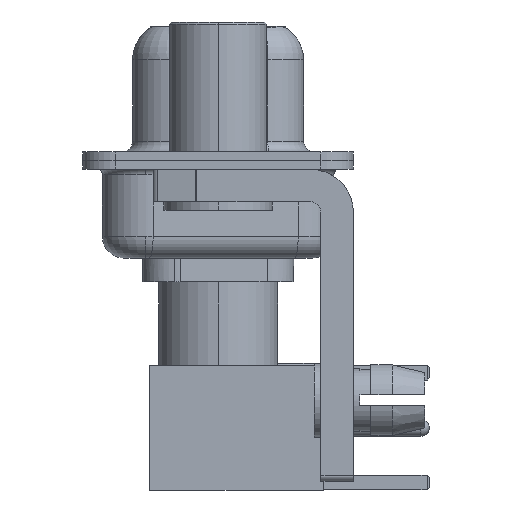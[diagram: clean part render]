
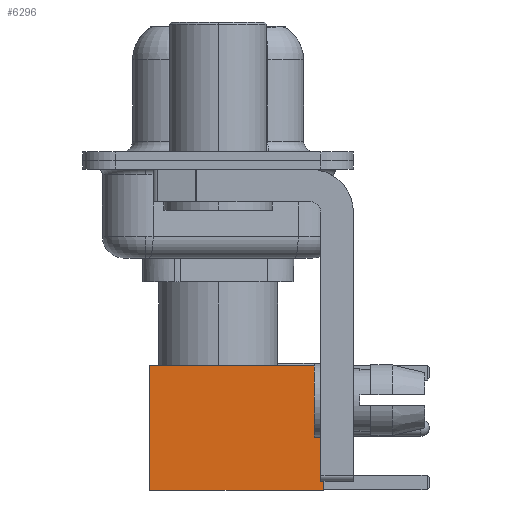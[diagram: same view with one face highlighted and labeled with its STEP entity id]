
A CAD part, left-side view. The second image highlights one B-rep face of the part: STEP entity #6296.
In plain terms, the highlighted face is planar.
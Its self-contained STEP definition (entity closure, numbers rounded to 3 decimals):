
#2625 = VECTOR ( 'NONE', #24853, 1000. ) ;
#3859 = LINE ( 'NONE', #10494, #13095 ) ;
#5786 = EDGE_CURVE ( 'NONE', #8243, #8651, #3859, .T. ) ;
#6296 = ADVANCED_FACE ( 'NONE', ( #19059 ), #22166, .T. ) ;
#7307 = VECTOR ( 'NONE', #13173, 1000. ) ;
#8243 = VERTEX_POINT ( 'NONE', #17881 ) ;
#8345 = EDGE_CURVE ( 'NONE', #23817, #8651, #9927, .T. ) ;
#8651 = VERTEX_POINT ( 'NONE', #23535 ) ;
#9121 = LINE ( 'NONE', #19712, #22267 ) ;
#9388 = DIRECTION ( 'NONE',  ( 0., 0., -1. ) ) ;
#9927 = LINE ( 'NONE', #11514, #2625 ) ;
#10494 = CARTESIAN_POINT ( 'NONE',  ( -2.875, 2.875, 0. ) ) ;
#10622 = VERTEX_POINT ( 'NONE', #17452 ) ;
#11108 = CARTESIAN_POINT ( 'NONE',  ( 2.875, 2.875, 0. ) ) ;
#11514 = CARTESIAN_POINT ( 'NONE',  ( 0., 2.875, 0. ) ) ;
#11802 = ORIENTED_EDGE ( 'NONE', *, *, #24969, .F. ) ;
#11872 = ORIENTED_EDGE ( 'NONE', *, *, #5786, .F. ) ;
#13095 = VECTOR ( 'NONE', #21382, 1000. ) ;
#13173 = DIRECTION ( 'NONE',  ( -1., 0., 0. ) ) ;
#13305 = DIRECTION ( 'NONE',  ( 0., 0., 1. ) ) ;
#13324 = CARTESIAN_POINT ( 'NONE',  ( 0., 2.875, 8. ) ) ;
#17452 = CARTESIAN_POINT ( 'NONE',  ( 2.875, 2.875, 8. ) ) ;
#17468 = ORIENTED_EDGE ( 'NONE', *, *, #8345, .T. ) ;
#17578 = DIRECTION ( 'NONE',  ( 0., 1., 0. ) ) ;
#17640 = EDGE_LOOP ( 'NONE', ( #24062, #17468, #11872, #11802 ) ) ;
#17881 = CARTESIAN_POINT ( 'NONE',  ( -2.875, 2.875, 8. ) ) ;
#19059 = FACE_OUTER_BOUND ( 'NONE', #17640, .T. ) ;
#19712 = CARTESIAN_POINT ( 'NONE',  ( 2.875, 2.875, 0. ) ) ;
#20883 = EDGE_CURVE ( 'NONE', #10622, #23817, #9121, .T. ) ;
#21382 = DIRECTION ( 'NONE',  ( 0., 0., -1. ) ) ;
#22166 = PLANE ( 'NONE',  #22288 ) ;
#22267 = VECTOR ( 'NONE', #9388, 1000. ) ;
#22288 = AXIS2_PLACEMENT_3D ( 'NONE', #27820, #17578, #13305 ) ;
#23535 = CARTESIAN_POINT ( 'NONE',  ( -2.875, 2.875, 0. ) ) ;
#23817 = VERTEX_POINT ( 'NONE', #11108 ) ;
#24062 = ORIENTED_EDGE ( 'NONE', *, *, #20883, .T. ) ;
#24853 = DIRECTION ( 'NONE',  ( -1., 0., 0. ) ) ;
#24969 = EDGE_CURVE ( 'NONE', #10622, #8243, #26360, .T. ) ;
#26360 = LINE ( 'NONE', #13324, #7307 ) ;
#27820 = CARTESIAN_POINT ( 'NONE',  ( 2.875, 2.875, 0. ) ) ;
